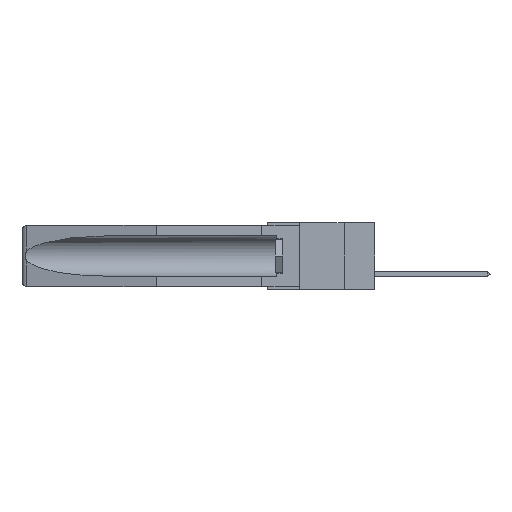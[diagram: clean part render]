
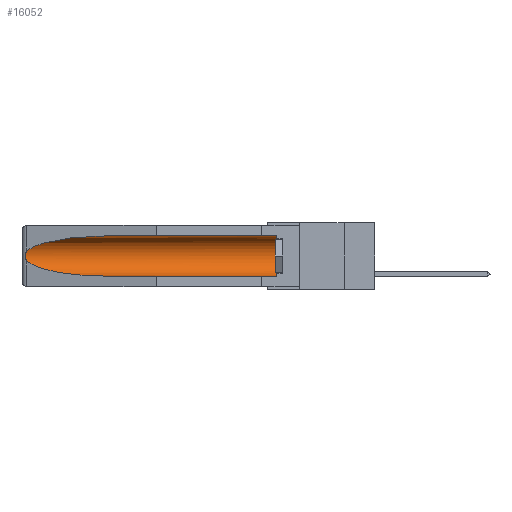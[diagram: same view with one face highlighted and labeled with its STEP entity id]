
A CAD part, left-side view. The second image highlights one B-rep face of the part: STEP entity #16052.
In plain terms, the highlighted cylindrical face has radius 2.857 mm (diameter 5.715 mm), a partial arc.
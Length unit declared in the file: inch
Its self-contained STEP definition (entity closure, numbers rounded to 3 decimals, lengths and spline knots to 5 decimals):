
#184 = DIRECTION ( 'NONE',  ( 0., 1., 0. ) ) ;
#523 = DIRECTION ( 'NONE',  ( 0., 0., 1. ) ) ;
#530 = CARTESIAN_POINT ( 'NONE',  ( 0.26597, 1.52961, -0.15275 ) ) ;
#789 = CARTESIAN_POINT ( 'NONE',  ( 0.26597, 1.5296, -0.19026 ) ) ;
#826 = DIRECTION ( 'NONE',  ( 0., 0., 1. ) ) ;
#1764 = ORIENTED_EDGE ( 'NONE', *, *, #4792, .F. ) ;
#1846 = CARTESIAN_POINT ( 'NONE',  ( 0.155, 0.126, -0.284 ) ) ;
#2725 = CARTESIAN_POINT ( 'NONE',  ( 0.26654, 1.53092, -0.15636 ) ) ;
#3840 = CARTESIAN_POINT ( 'NONE',  ( 0.21114, 1.30732, -0.284 ) ) ;
#4494 = ORIENTED_EDGE ( 'NONE', *, *, #23647, .T. ) ;
#4792 = EDGE_CURVE ( 'NONE', #11257, #5464, #18354, .T. ) ;
#5371 = LINE ( 'NONE', #21566, #22319 ) ;
#5464 = VERTEX_POINT ( 'NONE', #17614 ) ;
#5473 = EDGE_CURVE ( 'NONE', #15742, #9463, #24715, .T. ) ;
#6520 = CARTESIAN_POINT ( 'NONE',  ( 0.155, -0.30754, -0.284 ) ) ;
#7478 = CARTESIAN_POINT ( 'NONE',  ( 0.26537, 1.52718, -0.14972 ) ) ;
#7565 = CARTESIAN_POINT ( 'NONE',  ( 0.155, 1.07973, -0.059 ) ) ;
#8234 = AXIS2_PLACEMENT_3D ( 'NONE', #20727, #184, #523 ) ;
#8705 = CARTESIAN_POINT ( 'NONE',  ( 0.2673, 1.53269, -0.17917 ) ) ;
#9008 = DIRECTION ( 'NONE',  ( 0., -1., 0. ) ) ;
#9443 = CARTESIAN_POINT ( 'NONE',  ( 0.26537, 1.52718, -0.19328 ) ) ;
#9463 = VERTEX_POINT ( 'NONE', #13714 ) ;
#9912 = CARTESIAN_POINT ( 'NONE',  ( 0.25451, 1.48313, -0.24835 ) ) ;
#9945 = EDGE_CURVE ( 'NONE', #9463, #15716, #11617, .T. ) ;
#10251 = EDGE_CURVE ( 'NONE', #15716, #5464, #19426, .T. ) ;
#11013 = CARTESIAN_POINT ( 'NONE',  ( 0.155, 0.126, -0.1715 ) ) ;
#11257 = VERTEX_POINT ( 'NONE', #1846 ) ;
#11515 = CARTESIAN_POINT ( 'NONE',  ( 0.25451, 1.48313, -0.09465 ) ) ;
#11617 = B_SPLINE_CURVE_WITH_KNOTS ( 'NONE', 3,
 ( #12749, #530, #2725, #18928, #18849, #17148, #8705, #13082, #789, #12833 ),
 .UNSPECIFIED., .F., .F.,
 ( 4, 2, 2, 2, 4 ),
 ( 0., 0.00029, 0.00058, 0.00087, 0.00117 ),
 .UNSPECIFIED. ) ;
#12512 = CYLINDRICAL_SURFACE ( 'NONE', #8234, 0.1125 ) ;
#12749 = CARTESIAN_POINT ( 'NONE',  ( 0.26537, 1.52718, -0.14972 ) ) ;
#12833 = CARTESIAN_POINT ( 'NONE',  ( 0.26537, 1.52718, -0.19328 ) ) ;
#12839 = CIRCLE ( 'NONE', #16679, 0.1125 ) ;
#13082 = CARTESIAN_POINT ( 'NONE',  ( 0.26655, 1.53094, -0.18657 ) ) ;
#13083 = CARTESIAN_POINT ( 'NONE',  ( 0.155, 0.126, -0.059 ) ) ;
#13463 = CARTESIAN_POINT ( 'NONE',  ( 0.21114, 1.30732, -0.059 ) ) ;
#13485 = ORIENTED_EDGE ( 'NONE', *, *, #10251, .T. ) ;
#13714 = CARTESIAN_POINT ( 'NONE',  ( 0.26537, 1.52718, -0.14972 ) ) ;
#13751 = DIRECTION ( 'NONE',  ( 0., 1., 0. ) ) ;
#13861 = CARTESIAN_POINT ( 'NONE',  ( 0.26537, 1.52718, -0.19328 ) ) ;
#15716 = VERTEX_POINT ( 'NONE', #9443 ) ;
#15742 = VERTEX_POINT ( 'NONE', #7565 ) ;
#16052 = ADVANCED_FACE ( 'NONE', ( #16942 ), #12512, .F. ) ;
#16118 = ORIENTED_EDGE ( 'NONE', *, *, #9945, .T. ) ;
#16457 = VECTOR ( 'NONE', #20778, 39.37008 ) ;
#16679 = AXIS2_PLACEMENT_3D ( 'NONE', #11013, #9008, #826 ) ;
#16942 = FACE_OUTER_BOUND ( 'NONE', #25020, .T. ) ;
#17125 = ORIENTED_EDGE ( 'NONE', *, *, #5473, .T. ) ;
#17148 = CARTESIAN_POINT ( 'NONE',  ( 0.2675, 1.53308, -0.17534 ) ) ;
#17614 = CARTESIAN_POINT ( 'NONE',  ( 0.155, 1.07973, -0.284 ) ) ;
#17797 = ORIENTED_EDGE ( 'NONE', *, *, #23764, .T. ) ;
#17839 = VERTEX_POINT ( 'NONE', #13083 ) ;
#18354 = LINE ( 'NONE', #6520, #16457 ) ;
#18849 = CARTESIAN_POINT ( 'NONE',  ( 0.2675, 1.53308, -0.16763 ) ) ;
#18928 = CARTESIAN_POINT ( 'NONE',  ( 0.2673, 1.5327, -0.16383 ) ) ;
#19426 =( BOUNDED_CURVE ( )  B_SPLINE_CURVE ( 3, ( #13861, #9912, #3840, #20133 ),
 .UNSPECIFIED., .F., .F. ) 
 B_SPLINE_CURVE_WITH_KNOTS ( ( 4, 4 ),
 ( 0.1948, 1.5708 ),
 .UNSPECIFIED. ) 
 CURVE ( )  GEOMETRIC_REPRESENTATION_ITEM ( )  RATIONAL_B_SPLINE_CURVE ( ( 1., 0.848, 0.848, 1. ) ) 
 REPRESENTATION_ITEM ( '' )  );
#20133 = CARTESIAN_POINT ( 'NONE',  ( 0.155, 1.07973, -0.284 ) ) ;
#20727 = CARTESIAN_POINT ( 'NONE',  ( 0.155, -0.30754, -0.1715 ) ) ;
#20778 = DIRECTION ( 'NONE',  ( 0., 1., 0. ) ) ;
#21566 = CARTESIAN_POINT ( 'NONE',  ( 0.155, -0.30754, -0.059 ) ) ;
#21640 = CARTESIAN_POINT ( 'NONE',  ( 0.155, 1.07973, -0.059 ) ) ;
#22319 = VECTOR ( 'NONE', #13751, 39.37008 ) ;
#23647 = EDGE_CURVE ( 'NONE', #11257, #17839, #12839, .T. ) ;
#23764 = EDGE_CURVE ( 'NONE', #17839, #15742, #5371, .T. ) ;
#24715 =( BOUNDED_CURVE ( )  B_SPLINE_CURVE ( 3, ( #21640, #13463, #11515, #7478 ),
 .UNSPECIFIED., .F., .T. ) 
 B_SPLINE_CURVE_WITH_KNOTS ( ( 4, 4 ),
 ( 4.71239, 6.08839 ),
 .UNSPECIFIED. ) 
 CURVE ( )  GEOMETRIC_REPRESENTATION_ITEM ( )  RATIONAL_B_SPLINE_CURVE ( ( 1., 0.848, 0.848, 1. ) ) 
 REPRESENTATION_ITEM ( '' )  );
#25020 = EDGE_LOOP ( 'NONE', ( #17125, #16118, #13485, #1764, #4494, #17797 ) ) ;
